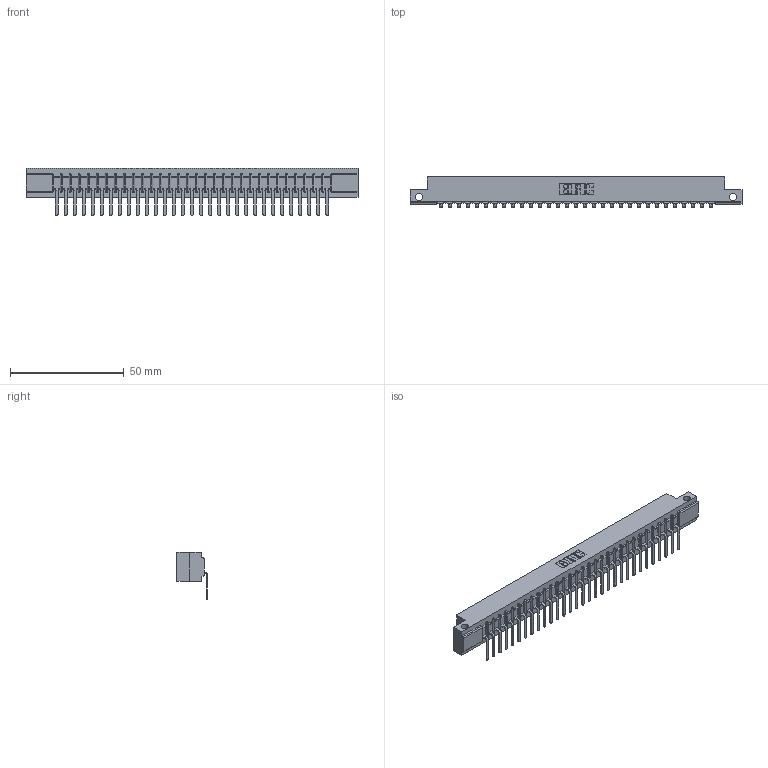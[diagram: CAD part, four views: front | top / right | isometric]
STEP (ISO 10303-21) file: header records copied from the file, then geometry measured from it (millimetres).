
FILE_DESCRIPTION (( 'STEP AP203' ), '1' );
FILE_NAME ('307-031-557-112.STEP', '2019-09-05T05:05:38', ( '' ), ( '' ), 'SwSTEP 2.0', 'SolidWorks 2016', '' );
FILE_SCHEMA (( 'CONFIG_CONTROL_DESIGN' ));
Length unit declared in the file: inch
Products named in the file (3): 307-290-002_557; 307-031-557-112; 307 Part_.128 Dia Side Mounting Holes
Assembly tree (32 placements, depth 2):
  307-031-557-112
    307 Part_.128 Dia Side Mounting Holes
    307-290-002_557  x31
Bounding box: 145.85 x 13.32 x 20.66 mm (x, y, z)
Volume: 15467 mm3; surface area: 19739.6 mm2
Topology: 32 solids, 32 shells, 2568 faces, 7887 edges, 5170 vertices
Faces by surface type: plane 1527, cylinder 977, sphere 64
Entity records: 28788 total; most frequent: CARTESIAN_POINT 4856, ORIENTED_EDGE 4846, DIRECTION 4723, EDGE_CURVE 2423, LINE 1849, VECTOR 1849, VERTEX_POINT 1570, AXIS2_PLACEMENT_3D 1437
